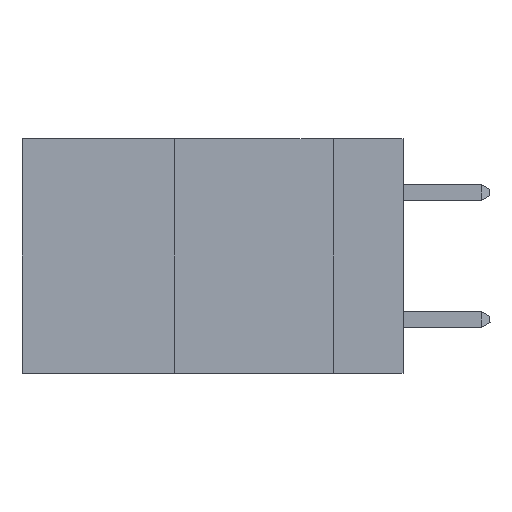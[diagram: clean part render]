
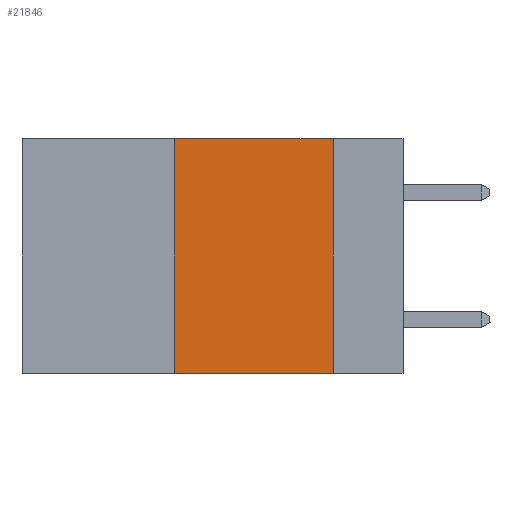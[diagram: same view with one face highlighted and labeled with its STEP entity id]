
A CAD part, left-side view. The second image highlights one B-rep face of the part: STEP entity #21846.
In plain terms, the highlighted planar face has unit normal (-1, 0, 0).
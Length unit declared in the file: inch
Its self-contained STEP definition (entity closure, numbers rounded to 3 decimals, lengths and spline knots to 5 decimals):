
#614 = CARTESIAN_POINT ( 'NONE',  ( 0., 0.36, 0. ) ) ;
#735 = FACE_OUTER_BOUND ( 'NONE', #4067, .T. ) ;
#1311 = CARTESIAN_POINT ( 'NONE',  ( 0., 0.6, -0.37 ) ) ;
#1507 = AXIS2_PLACEMENT_3D ( 'NONE', #17345, #7380, #21358 ) ;
#2597 = LINE ( 'NONE', #5079, #7390 ) ;
#3572 = VERTEX_POINT ( 'NONE', #24235 ) ;
#3908 = LINE ( 'NONE', #18838, #9286 ) ;
#4067 = EDGE_LOOP ( 'NONE', ( #19855, #13915, #5787, #15814 ) ) ;
#4818 = DIRECTION ( 'NONE',  ( 0., 0., -1. ) ) ;
#5079 = CARTESIAN_POINT ( 'NONE',  ( 0., 0.11, 0. ) ) ;
#5787 = ORIENTED_EDGE ( 'NONE', *, *, #15836, .F. ) ;
#5859 = EDGE_CURVE ( 'NONE', #10863, #7742, #3908, .T. ) ;
#5937 = EDGE_CURVE ( 'NONE', #7742, #3572, #2597, .T. ) ;
#6114 = VECTOR ( 'NONE', #22779, 39.37008 ) ;
#7380 = DIRECTION ( 'NONE',  ( 1., 0., 0. ) ) ;
#7390 = VECTOR ( 'NONE', #4818, 39.37008 ) ;
#7621 = CARTESIAN_POINT ( 'NONE',  ( 0., 0.11, 0. ) ) ;
#7742 = VERTEX_POINT ( 'NONE', #7621 ) ;
#8544 = VERTEX_POINT ( 'NONE', #22067 ) ;
#9286 = VECTOR ( 'NONE', #15711, 39.37008 ) ;
#10490 = EDGE_CURVE ( 'NONE', #8544, #3572, #14631, .T. ) ;
#10863 = VERTEX_POINT ( 'NONE', #18488 ) ;
#11346 = PLANE ( 'NONE',  #1507 ) ;
#11467 = LINE ( 'NONE', #614, #6114 ) ;
#13915 = ORIENTED_EDGE ( 'NONE', *, *, #5859, .F. ) ;
#14631 = LINE ( 'NONE', #1311, #15255 ) ;
#15255 = VECTOR ( 'NONE', #23342, 39.37008 ) ;
#15711 = DIRECTION ( 'NONE',  ( 0., -1., 0. ) ) ;
#15814 = ORIENTED_EDGE ( 'NONE', *, *, #10490, .T. ) ;
#15836 = EDGE_CURVE ( 'NONE', #8544, #10863, #11467, .T. ) ;
#17345 = CARTESIAN_POINT ( 'NONE',  ( 0., 0.6, 0. ) ) ;
#18488 = CARTESIAN_POINT ( 'NONE',  ( 0., 0.36, 0. ) ) ;
#18838 = CARTESIAN_POINT ( 'NONE',  ( 0., 0.6, 0. ) ) ;
#19855 = ORIENTED_EDGE ( 'NONE', *, *, #5937, .F. ) ;
#21358 = DIRECTION ( 'NONE',  ( 0., 0., -1. ) ) ;
#21846 = ADVANCED_FACE ( 'NONE', ( #735 ), #11346, .F. ) ;
#22067 = CARTESIAN_POINT ( 'NONE',  ( 0., 0.36, -0.37 ) ) ;
#22779 = DIRECTION ( 'NONE',  ( 0., 0., 1. ) ) ;
#23342 = DIRECTION ( 'NONE',  ( 0., -1., 0. ) ) ;
#24235 = CARTESIAN_POINT ( 'NONE',  ( 0., 0.11, -0.37 ) ) ;
